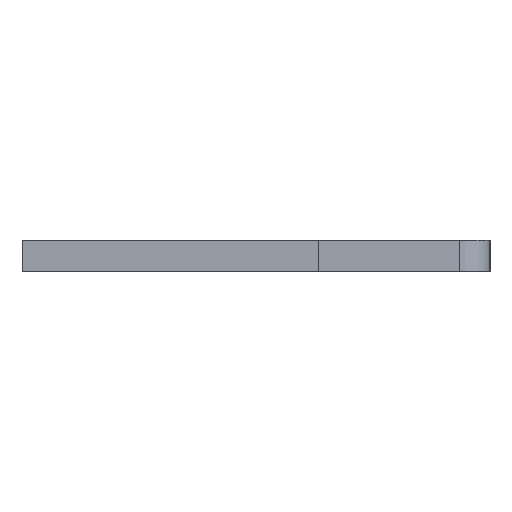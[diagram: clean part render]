
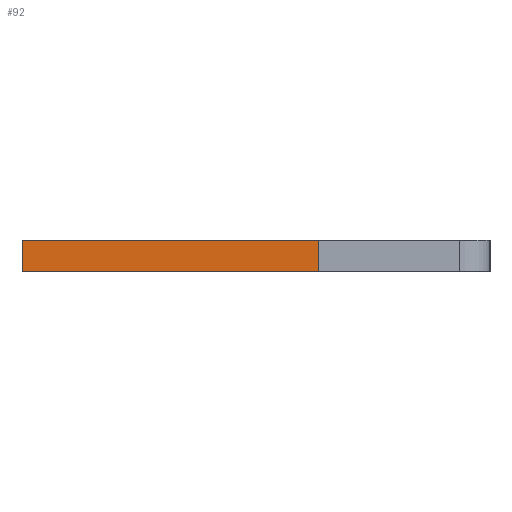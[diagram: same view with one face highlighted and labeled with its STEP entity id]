
A CAD part, left-side view. The second image highlights one B-rep face of the part: STEP entity #92.
In plain terms, the highlighted face is planar.
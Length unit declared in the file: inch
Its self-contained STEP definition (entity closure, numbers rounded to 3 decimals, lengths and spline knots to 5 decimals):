
#37 = DIRECTION ( 'NONE',  ( 0., 1., 0. ) ) ;
#57 = VERTEX_POINT ( 'NONE', #349 ) ;
#70 = VECTOR ( 'NONE', #37, 39.37008 ) ;
#79 = ORIENTED_EDGE ( 'NONE', *, *, #702, .F. ) ;
#86 = LINE ( 'NONE', #838, #168 ) ;
#92 = ADVANCED_FACE ( 'NONE', ( #798 ), #1045, .F. ) ;
#126 = CARTESIAN_POINT ( 'NONE',  ( 0.01, -0.04, -0.04 ) ) ;
#163 = EDGE_CURVE ( 'NONE', #481, #955, #86, .T. ) ;
#168 = VECTOR ( 'NONE', #192, 39.37008 ) ;
#192 = DIRECTION ( 'NONE',  ( -1., 0., 0. ) ) ;
#273 = DIRECTION ( 'NONE',  ( 1., 0., 0. ) ) ;
#309 = VECTOR ( 'NONE', #1084, 39.37008 ) ;
#336 = DIRECTION ( 'NONE',  ( -1., 0., 0. ) ) ;
#349 = CARTESIAN_POINT ( 'NONE',  ( -0.01, -0.04, -0.04 ) ) ;
#383 = CARTESIAN_POINT ( 'NONE',  ( 0.01, 0.15, -0.04 ) ) ;
#403 = ORIENTED_EDGE ( 'NONE', *, *, #1034, .T. ) ;
#426 = CARTESIAN_POINT ( 'NONE',  ( 0.01, -0.04, -0.04 ) ) ;
#481 = VERTEX_POINT ( 'NONE', #383 ) ;
#491 = ORIENTED_EDGE ( 'NONE', *, *, #577, .T. ) ;
#516 = EDGE_LOOP ( 'NONE', ( #491, #962, #79, #403 ) ) ;
#524 = LINE ( 'NONE', #1014, #70 ) ;
#577 = EDGE_CURVE ( 'NONE', #57, #955, #768, .T. ) ;
#600 = AXIS2_PLACEMENT_3D ( 'NONE', #611, #993, #273 ) ;
#611 = CARTESIAN_POINT ( 'NONE',  ( 0.01, 0.15, -0.04 ) ) ;
#666 = VERTEX_POINT ( 'NONE', #126 ) ;
#692 = LINE ( 'NONE', #426, #773 ) ;
#702 = EDGE_CURVE ( 'NONE', #666, #481, #524, .T. ) ;
#768 = LINE ( 'NONE', #1006, #309 ) ;
#773 = VECTOR ( 'NONE', #336, 39.37008 ) ;
#776 = CARTESIAN_POINT ( 'NONE',  ( -0.01, 0.15, -0.04 ) ) ;
#798 = FACE_OUTER_BOUND ( 'NONE', #516, .T. ) ;
#838 = CARTESIAN_POINT ( 'NONE',  ( 0.01, 0.15, -0.04 ) ) ;
#955 = VERTEX_POINT ( 'NONE', #776 ) ;
#962 = ORIENTED_EDGE ( 'NONE', *, *, #163, .F. ) ;
#993 = DIRECTION ( 'NONE',  ( 0., 0., 1. ) ) ;
#1006 = CARTESIAN_POINT ( 'NONE',  ( -0.01, 0.15, -0.04 ) ) ;
#1014 = CARTESIAN_POINT ( 'NONE',  ( 0.01, 0.15, -0.04 ) ) ;
#1034 = EDGE_CURVE ( 'NONE', #666, #57, #692, .T. ) ;
#1045 = PLANE ( 'NONE',  #600 ) ;
#1084 = DIRECTION ( 'NONE',  ( 0., 1., 0. ) ) ;
